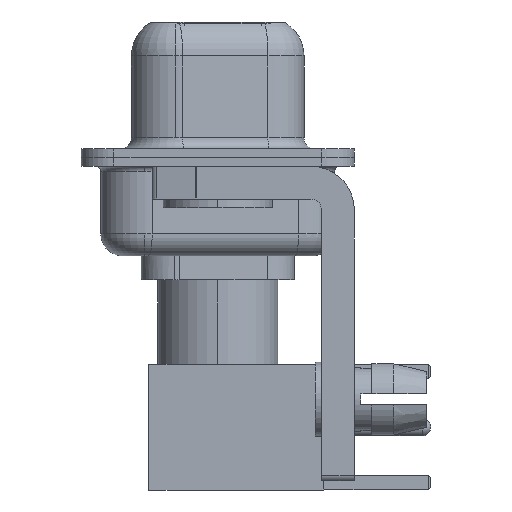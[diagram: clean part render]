
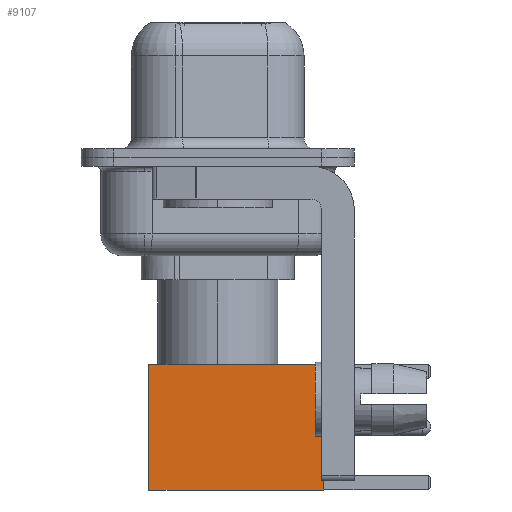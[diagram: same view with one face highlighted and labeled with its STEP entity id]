
A CAD part, left-side view. The second image highlights one B-rep face of the part: STEP entity #9107.
In plain terms, the highlighted face is planar.
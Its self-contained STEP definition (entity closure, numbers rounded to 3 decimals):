
#233 = CARTESIAN_POINT ( 'NONE',  ( -2.875, 2.875, 0. ) ) ;
#607 = VECTOR ( 'NONE', #4524, 1000. ) ;
#777 = EDGE_CURVE ( 'NONE', #12549, #14320, #9288, .T. ) ;
#975 = ORIENTED_EDGE ( 'NONE', *, *, #777, .T. ) ;
#989 = EDGE_CURVE ( 'NONE', #16206, #12549, #3589, .T. ) ;
#1322 = CARTESIAN_POINT ( 'NONE',  ( 0., 2.875, 0. ) ) ;
#1640 = VECTOR ( 'NONE', #10223, 1000. ) ;
#3291 = DIRECTION ( 'NONE',  ( 0., 1., 0. ) ) ;
#3589 = LINE ( 'NONE', #17308, #15456 ) ;
#4521 = CARTESIAN_POINT ( 'NONE',  ( -2.875, 2.875, 0. ) ) ;
#4524 = DIRECTION ( 'NONE',  ( 0., 0., -1. ) ) ;
#5271 = EDGE_CURVE ( 'NONE', #14750, #14320, #11208, .T. ) ;
#6843 = DIRECTION ( 'NONE',  ( -1., 0., 0. ) ) ;
#7101 = ORIENTED_EDGE ( 'NONE', *, *, #5271, .F. ) ;
#8011 = CARTESIAN_POINT ( 'NONE',  ( 2.875, 2.875, 0. ) ) ;
#8498 = CARTESIAN_POINT ( 'NONE',  ( 0., 2.875, 8. ) ) ;
#9107 = ADVANCED_FACE ( 'NONE', ( #14076 ), #11260, .T. ) ;
#9286 = EDGE_LOOP ( 'NONE', ( #12219, #975, #7101, #16055 ) ) ;
#9288 = LINE ( 'NONE', #1322, #17195 ) ;
#9897 = DIRECTION ( 'NONE',  ( 0., 0., 1. ) ) ;
#10223 = DIRECTION ( 'NONE',  ( -1., 0., 0. ) ) ;
#11208 = LINE ( 'NONE', #233, #607 ) ;
#11260 = PLANE ( 'NONE',  #14495 ) ;
#11587 = LINE ( 'NONE', #8498, #1640 ) ;
#11912 = DIRECTION ( 'NONE',  ( 0., 0., -1. ) ) ;
#12219 = ORIENTED_EDGE ( 'NONE', *, *, #989, .T. ) ;
#12549 = VERTEX_POINT ( 'NONE', #8011 ) ;
#12574 = CARTESIAN_POINT ( 'NONE',  ( -2.875, 2.875, 8. ) ) ;
#13998 = CARTESIAN_POINT ( 'NONE',  ( 2.875, 2.875, 8. ) ) ;
#14076 = FACE_OUTER_BOUND ( 'NONE', #9286, .T. ) ;
#14320 = VERTEX_POINT ( 'NONE', #4521 ) ;
#14495 = AXIS2_PLACEMENT_3D ( 'NONE', #16822, #3291, #9897 ) ;
#14750 = VERTEX_POINT ( 'NONE', #12574 ) ;
#15456 = VECTOR ( 'NONE', #11912, 1000. ) ;
#16055 = ORIENTED_EDGE ( 'NONE', *, *, #17167, .F. ) ;
#16206 = VERTEX_POINT ( 'NONE', #13998 ) ;
#16822 = CARTESIAN_POINT ( 'NONE',  ( 2.875, 2.875, 0. ) ) ;
#17167 = EDGE_CURVE ( 'NONE', #16206, #14750, #11587, .T. ) ;
#17195 = VECTOR ( 'NONE', #6843, 1000. ) ;
#17308 = CARTESIAN_POINT ( 'NONE',  ( 2.875, 2.875, 0. ) ) ;
